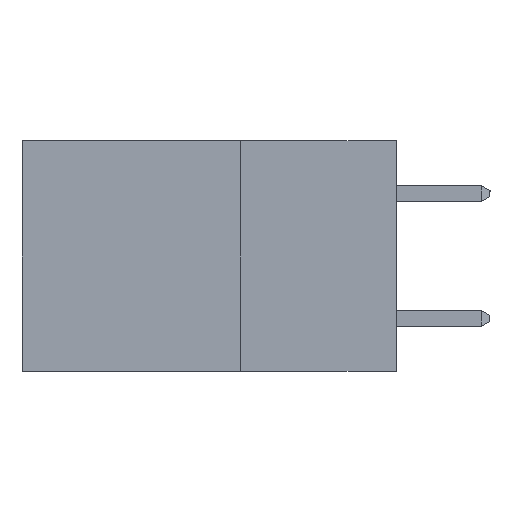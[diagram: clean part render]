
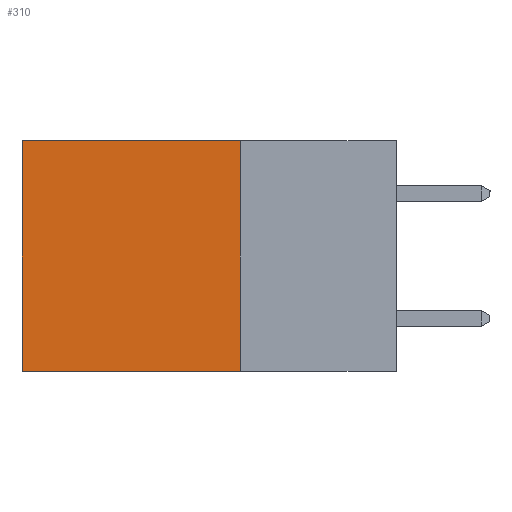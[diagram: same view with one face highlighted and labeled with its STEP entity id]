
A CAD part, left-side view. The second image highlights one B-rep face of the part: STEP entity #310.
In plain terms, the highlighted planar face has unit normal (-1, 0, 0).
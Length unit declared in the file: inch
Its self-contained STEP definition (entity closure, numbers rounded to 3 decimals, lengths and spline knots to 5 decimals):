
#145 = CARTESIAN_POINT ( 'NONE',  ( 0.2615, 0.25, -0.37 ) ) ;
#310 = ADVANCED_FACE ( 'NONE', ( #8593 ), #11551, .F. ) ;
#958 = AXIS2_PLACEMENT_3D ( 'NONE', #145, #1379, #2331 ) ;
#1179 = ORIENTED_EDGE ( 'NONE', *, *, #1785, .F. ) ;
#1379 = DIRECTION ( 'NONE',  ( 1., 0., 0. ) ) ;
#1743 = LINE ( 'NONE', #10845, #10337 ) ;
#1785 = EDGE_CURVE ( 'NONE', #7220, #6745, #2544, .T. ) ;
#2331 = DIRECTION ( 'NONE',  ( 0., 0., -1. ) ) ;
#2544 = LINE ( 'NONE', #2805, #3292 ) ;
#2592 = CARTESIAN_POINT ( 'NONE',  ( 0.2615, 0.25, 0. ) ) ;
#2805 = CARTESIAN_POINT ( 'NONE',  ( 0.2615, 0.25, -0.37 ) ) ;
#3292 = VECTOR ( 'NONE', #6835, 39.37008 ) ;
#3639 = VERTEX_POINT ( 'NONE', #2592 ) ;
#4164 = EDGE_LOOP ( 'NONE', ( #4276, #1179, #6635, #11903 ) ) ;
#4276 = ORIENTED_EDGE ( 'NONE', *, *, #5903, .T. ) ;
#4852 = DIRECTION ( 'NONE',  ( 0., 0., -1. ) ) ;
#5797 = CARTESIAN_POINT ( 'NONE',  ( 0.2615, 0.25, 0. ) ) ;
#5823 = VECTOR ( 'NONE', #12881, 39.37008 ) ;
#5903 = EDGE_CURVE ( 'NONE', #8630, #6745, #1743, .T. ) ;
#5952 = EDGE_CURVE ( 'NONE', #3639, #8630, #6873, .T. ) ;
#6635 = ORIENTED_EDGE ( 'NONE', *, *, #10511, .F. ) ;
#6745 = VERTEX_POINT ( 'NONE', #10863 ) ;
#6835 = DIRECTION ( 'NONE',  ( 0., 1., 0. ) ) ;
#6873 = LINE ( 'NONE', #5797, #5823 ) ;
#7220 = VERTEX_POINT ( 'NONE', #11927 ) ;
#8243 = VECTOR ( 'NONE', #10435, 39.37008 ) ;
#8289 = CARTESIAN_POINT ( 'NONE',  ( 0.2615, 0.25, -0.37 ) ) ;
#8593 = FACE_OUTER_BOUND ( 'NONE', #4164, .T. ) ;
#8630 = VERTEX_POINT ( 'NONE', #13153 ) ;
#10337 = VECTOR ( 'NONE', #4852, 39.37008 ) ;
#10435 = DIRECTION ( 'NONE',  ( 0., 0., -1. ) ) ;
#10511 = EDGE_CURVE ( 'NONE', #3639, #7220, #10565, .T. ) ;
#10565 = LINE ( 'NONE', #8289, #8243 ) ;
#10845 = CARTESIAN_POINT ( 'NONE',  ( 0.2615, 0.6, -0.37 ) ) ;
#10863 = CARTESIAN_POINT ( 'NONE',  ( 0.2615, 0.6, -0.37 ) ) ;
#11551 = PLANE ( 'NONE',  #958 ) ;
#11903 = ORIENTED_EDGE ( 'NONE', *, *, #5952, .T. ) ;
#11927 = CARTESIAN_POINT ( 'NONE',  ( 0.2615, 0.25, -0.37 ) ) ;
#12881 = DIRECTION ( 'NONE',  ( 0., 1., 0. ) ) ;
#13153 = CARTESIAN_POINT ( 'NONE',  ( 0.2615, 0.6, 0. ) ) ;
